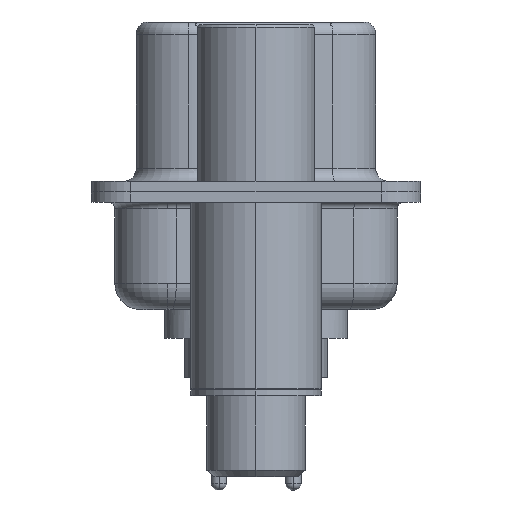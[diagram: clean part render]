
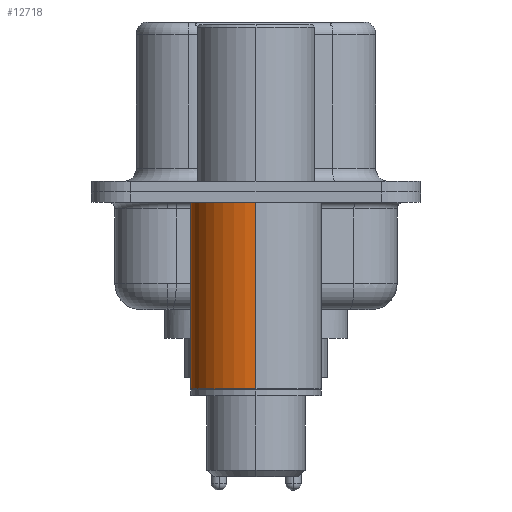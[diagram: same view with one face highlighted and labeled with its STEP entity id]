
A CAD part, left-side view. The second image highlights one B-rep face of the part: STEP entity #12718.
In plain terms, the highlighted cylindrical face has radius 2.5 mm (diameter 5 mm), a partial arc.
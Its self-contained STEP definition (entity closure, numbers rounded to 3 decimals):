
#76 = VERTEX_POINT ( 'NONE', #1553 ) ;
#856 = ORIENTED_EDGE ( 'NONE', *, *, #6015, .F. ) ;
#1553 = CARTESIAN_POINT ( 'NONE',  ( -2.5, 0., -0.4 ) ) ;
#1859 = VERTEX_POINT ( 'NONE', #23070 ) ;
#3398 = DIRECTION ( 'NONE',  ( 0., 0., 1. ) ) ;
#3692 = ORIENTED_EDGE ( 'NONE', *, *, #8806, .F. ) ;
#4277 = CARTESIAN_POINT ( 'NONE',  ( 0., 0., 0.581 ) ) ;
#5453 = VERTEX_POINT ( 'NONE', #14137 ) ;
#5626 = DIRECTION ( 'NONE',  ( 1., 0., 0. ) ) ;
#6015 = EDGE_CURVE ( 'NONE', #5453, #76, #20966, .T. ) ;
#6222 = DIRECTION ( 'NONE',  ( 0., 0., 1. ) ) ;
#6230 = VECTOR ( 'NONE', #3398, 1000. ) ;
#8020 = VECTOR ( 'NONE', #20541, 1000. ) ;
#8806 = EDGE_CURVE ( 'NONE', #13516, #5453, #18145, .T. ) ;
#9239 = CARTESIAN_POINT ( 'NONE',  ( -2.5, 0., 0.581 ) ) ;
#11740 = DIRECTION ( 'NONE',  ( 0., 0., 1. ) ) ;
#12371 = EDGE_CURVE ( 'NONE', #13516, #1859, #15702, .T. ) ;
#12718 = ADVANCED_FACE ( 'NONE', ( #20398 ), #14812, .T. ) ;
#13191 = DIRECTION ( 'NONE',  ( 0., 0., 1. ) ) ;
#13251 = CARTESIAN_POINT ( 'NONE',  ( 0., 0., -0.4 ) ) ;
#13516 = VERTEX_POINT ( 'NONE', #22481 ) ;
#14086 = EDGE_LOOP ( 'NONE', ( #24892, #23882, #856, #3692 ) ) ;
#14137 = CARTESIAN_POINT ( 'NONE',  ( 2.5, 0., -0.4 ) ) ;
#14812 = CYLINDRICAL_SURFACE ( 'NONE', #24639, 2.5 ) ;
#15702 = CIRCLE ( 'NONE', #17387, 2.5 ) ;
#17387 = AXIS2_PLACEMENT_3D ( 'NONE', #23078, #11740, #25041 ) ;
#17777 = AXIS2_PLACEMENT_3D ( 'NONE', #13251, #13191, #5626 ) ;
#18145 = LINE ( 'NONE', #22918, #8020 ) ;
#20398 = FACE_OUTER_BOUND ( 'NONE', #14086, .T. ) ;
#20541 = DIRECTION ( 'NONE',  ( 0., 0., 1. ) ) ;
#20886 = LINE ( 'NONE', #9239, #6230 ) ;
#20966 = CIRCLE ( 'NONE', #17777, 2.5 ) ;
#21057 = EDGE_CURVE ( 'NONE', #1859, #76, #20886, .T. ) ;
#21501 = DIRECTION ( 'NONE',  ( 1., 0., 0. ) ) ;
#22481 = CARTESIAN_POINT ( 'NONE',  ( 2.5, 0., -7.525 ) ) ;
#22918 = CARTESIAN_POINT ( 'NONE',  ( 2.5, 0., 0.581 ) ) ;
#23070 = CARTESIAN_POINT ( 'NONE',  ( -2.5, 0., -7.525 ) ) ;
#23078 = CARTESIAN_POINT ( 'NONE',  ( 0., 0., -7.525 ) ) ;
#23882 = ORIENTED_EDGE ( 'NONE', *, *, #21057, .T. ) ;
#24639 = AXIS2_PLACEMENT_3D ( 'NONE', #4277, #6222, #21501 ) ;
#24892 = ORIENTED_EDGE ( 'NONE', *, *, #12371, .T. ) ;
#25041 = DIRECTION ( 'NONE',  ( 1., 0., 0. ) ) ;
